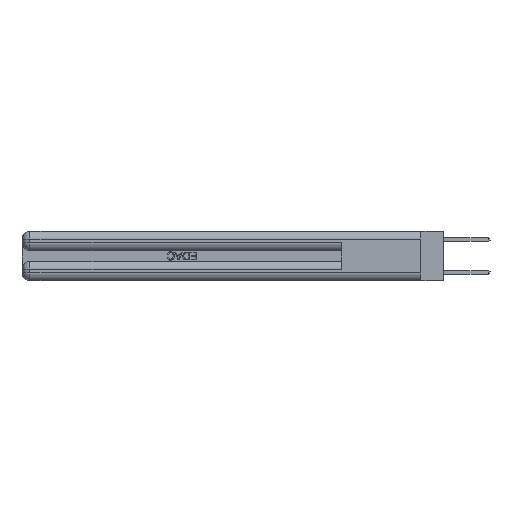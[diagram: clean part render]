
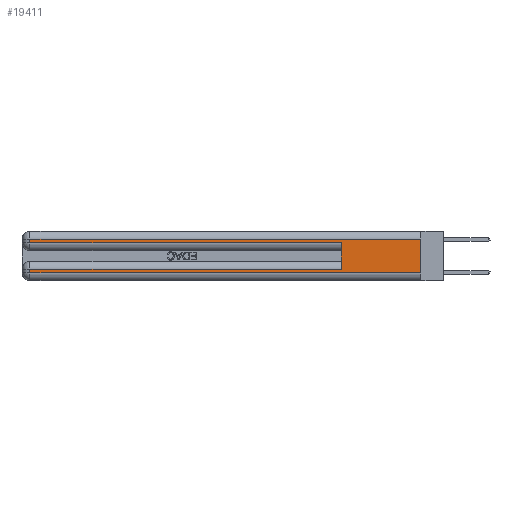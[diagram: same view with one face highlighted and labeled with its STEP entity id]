
A CAD part, left-side view. The second image highlights one B-rep face of the part: STEP entity #19411.
In plain terms, the highlighted planar face has unit normal (-1, 0, 0).
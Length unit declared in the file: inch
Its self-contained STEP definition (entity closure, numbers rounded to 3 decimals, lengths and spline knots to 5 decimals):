
#47 = VERTEX_POINT ( 'NONE', #124 ) ;
#124 = CARTESIAN_POINT ( 'NONE',  ( 0., 0., 0.06 ) ) ;
#434 = CARTESIAN_POINT ( 'NONE',  ( 0., 2.94, 0.37 ) ) ;
#1717 = CARTESIAN_POINT ( 'NONE',  ( 0., 0., 0.37 ) ) ;
#1796 = LINE ( 'NONE', #1978, #34985 ) ;
#1845 = CARTESIAN_POINT ( 'NONE',  ( 0., 0.6, 0.145 ) ) ;
#1978 = CARTESIAN_POINT ( 'NONE',  ( 0., 0., 0.37 ) ) ;
#2287 = EDGE_CURVE ( 'NONE', #18247, #16007, #24218, .T. ) ;
#3335 = CARTESIAN_POINT ( 'NONE',  ( 0., 0., 0.31 ) ) ;
#3624 = EDGE_CURVE ( 'NONE', #28480, #23211, #34738, .T. ) ;
#5348 = EDGE_CURVE ( 'NONE', #23211, #47, #26024, .T. ) ;
#5825 = VECTOR ( 'NONE', #6104, 39.37008 ) ;
#5930 = VECTOR ( 'NONE', #7383, 39.37008 ) ;
#6104 = DIRECTION ( 'NONE',  ( 0., -1., 0. ) ) ;
#7383 = DIRECTION ( 'NONE',  ( 0., 1., 0. ) ) ;
#8633 = DIRECTION ( 'NONE',  ( 0., 0., -1. ) ) ;
#10147 = EDGE_CURVE ( 'NONE', #13427, #33174, #16814, .T. ) ;
#11089 = VECTOR ( 'NONE', #8633, 39.37008 ) ;
#11933 = ORIENTED_EDGE ( 'NONE', *, *, #2287, .F. ) ;
#12125 = ORIENTED_EDGE ( 'NONE', *, *, #35505, .T. ) ;
#13427 = VERTEX_POINT ( 'NONE', #36673 ) ;
#14368 = CARTESIAN_POINT ( 'NONE',  ( 0., 0., 0.31 ) ) ;
#14388 = DIRECTION ( 'NONE',  ( 0., 0., -1. ) ) ;
#15416 = DIRECTION ( 'NONE',  ( 0., 0., -1. ) ) ;
#15883 = FACE_OUTER_BOUND ( 'NONE', #33819, .T. ) ;
#16007 = VERTEX_POINT ( 'NONE', #22954 ) ;
#16189 = ORIENTED_EDGE ( 'NONE', *, *, #5348, .T. ) ;
#16814 = LINE ( 'NONE', #28371, #32758 ) ;
#18247 = VERTEX_POINT ( 'NONE', #35999 ) ;
#18730 = LINE ( 'NONE', #27677, #5930 ) ;
#19411 = ADVANCED_FACE ( 'NONE', ( #15883 ), #23912, .F. ) ;
#20051 = ORIENTED_EDGE ( 'NONE', *, *, #24823, .F. ) ;
#21160 = ORIENTED_EDGE ( 'NONE', *, *, #10147, .T. ) ;
#21913 = CARTESIAN_POINT ( 'NONE',  ( 0., 2.94, 0.06 ) ) ;
#22637 = CARTESIAN_POINT ( 'NONE',  ( 0., 2.94, 0.085 ) ) ;
#22954 = CARTESIAN_POINT ( 'NONE',  ( 0., 0.6, 0.285 ) ) ;
#23000 = VERTEX_POINT ( 'NONE', #3335 ) ;
#23190 = CARTESIAN_POINT ( 'NONE',  ( 0., 0., 0.285 ) ) ;
#23211 = VERTEX_POINT ( 'NONE', #21913 ) ;
#23741 = DIRECTION ( 'NONE',  ( 0., -1., 0. ) ) ;
#23912 = PLANE ( 'NONE',  #36453 ) ;
#24218 = LINE ( 'NONE', #1845, #25632 ) ;
#24823 = EDGE_CURVE ( 'NONE', #23000, #47, #1796, .T. ) ;
#25632 = VECTOR ( 'NONE', #30019, 39.37008 ) ;
#25733 = DIRECTION ( 'NONE',  ( 0., 1., 0. ) ) ;
#26024 = LINE ( 'NONE', #28837, #5825 ) ;
#26038 = ORIENTED_EDGE ( 'NONE', *, *, #26188, .T. ) ;
#26188 = EDGE_CURVE ( 'NONE', #23000, #13427, #28718, .T. ) ;
#27677 = CARTESIAN_POINT ( 'NONE',  ( 0., 0., 0.085 ) ) ;
#27739 = ORIENTED_EDGE ( 'NONE', *, *, #29724, .T. ) ;
#28371 = CARTESIAN_POINT ( 'NONE',  ( 0., 2.94, 0.37 ) ) ;
#28480 = VERTEX_POINT ( 'NONE', #22637 ) ;
#28718 = LINE ( 'NONE', #14368, #30153 ) ;
#28837 = CARTESIAN_POINT ( 'NONE',  ( 0., 0., 0.06 ) ) ;
#29724 = EDGE_CURVE ( 'NONE', #18247, #28480, #18730, .T. ) ;
#30019 = DIRECTION ( 'NONE',  ( 0., 0., 1. ) ) ;
#30153 = VECTOR ( 'NONE', #25733, 39.37008 ) ;
#30421 = DIRECTION ( 'NONE',  ( 1., 0., 0. ) ) ;
#32097 = CARTESIAN_POINT ( 'NONE',  ( 0., 2.94, 0.285 ) ) ;
#32616 = ORIENTED_EDGE ( 'NONE', *, *, #3624, .T. ) ;
#32674 = DIRECTION ( 'NONE',  ( 0., 0., -1. ) ) ;
#32758 = VECTOR ( 'NONE', #14388, 39.37008 ) ;
#33174 = VERTEX_POINT ( 'NONE', #32097 ) ;
#33819 = EDGE_LOOP ( 'NONE', ( #20051, #26038, #21160, #12125, #11933, #27739, #32616, #16189 ) ) ;
#34267 = VECTOR ( 'NONE', #23741, 39.37008 ) ;
#34565 = LINE ( 'NONE', #23190, #34267 ) ;
#34738 = LINE ( 'NONE', #434, #11089 ) ;
#34985 = VECTOR ( 'NONE', #15416, 39.37008 ) ;
#35505 = EDGE_CURVE ( 'NONE', #33174, #16007, #34565, .T. ) ;
#35999 = CARTESIAN_POINT ( 'NONE',  ( 0., 0.6, 0.085 ) ) ;
#36453 = AXIS2_PLACEMENT_3D ( 'NONE', #1717, #30421, #32674 ) ;
#36673 = CARTESIAN_POINT ( 'NONE',  ( 0., 2.94, 0.31 ) ) ;
